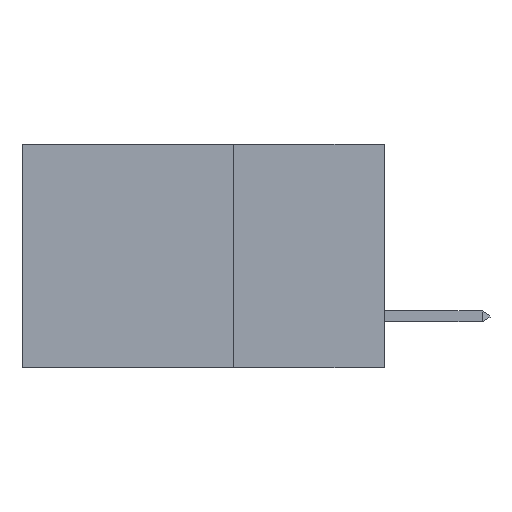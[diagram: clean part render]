
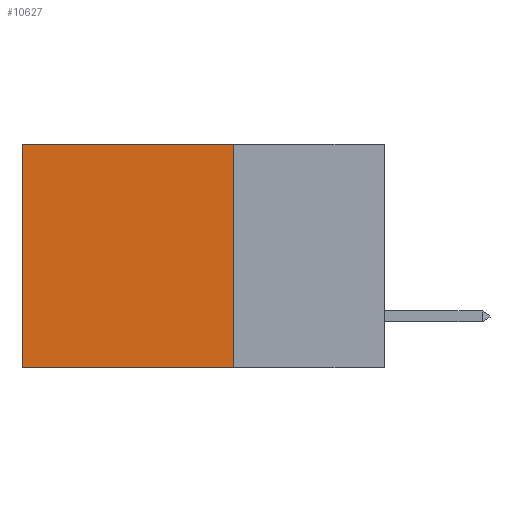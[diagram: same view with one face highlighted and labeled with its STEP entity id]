
A CAD part, left-side view. The second image highlights one B-rep face of the part: STEP entity #10627.
In plain terms, the highlighted planar face has unit normal (-1, 0, 0).
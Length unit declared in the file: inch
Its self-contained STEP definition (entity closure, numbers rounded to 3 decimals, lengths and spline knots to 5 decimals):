
#1636 = DIRECTION ( 'NONE',  ( 0., 0., -1. ) ) ;
#2250 = LINE ( 'NONE', #33708, #26084 ) ;
#4461 = EDGE_CURVE ( 'NONE', #18445, #30422, #2250, .T. ) ;
#4537 = ORIENTED_EDGE ( 'NONE', *, *, #19035, .T. ) ;
#8323 = CARTESIAN_POINT ( 'NONE',  ( 0.2875, 0.6, 0. ) ) ;
#9995 = DIRECTION ( 'NONE',  ( 0., 0., -1. ) ) ;
#10439 = EDGE_CURVE ( 'NONE', #30422, #24059, #21062, .T. ) ;
#10545 = PLANE ( 'NONE',  #28321 ) ;
#10627 = ADVANCED_FACE ( 'NONE', ( #14485 ), #10545, .F. ) ;
#12079 = ORIENTED_EDGE ( 'NONE', *, *, #4461, .F. ) ;
#12773 = DIRECTION ( 'NONE',  ( 0., 1., 0. ) ) ;
#12940 = EDGE_CURVE ( 'NONE', #21688, #24059, #29257, .T. ) ;
#14485 = FACE_OUTER_BOUND ( 'NONE', #36721, .T. ) ;
#15905 = ORIENTED_EDGE ( 'NONE', *, *, #12940, .T. ) ;
#18445 = VERTEX_POINT ( 'NONE', #25985 ) ;
#18540 = ORIENTED_EDGE ( 'NONE', *, *, #10439, .F. ) ;
#19035 = EDGE_CURVE ( 'NONE', #18445, #21688, #29015, .T. ) ;
#19536 = DIRECTION ( 'NONE',  ( 1., 0., 0. ) ) ;
#20107 = VECTOR ( 'NONE', #12773, 39.37008 ) ;
#20172 = VECTOR ( 'NONE', #37490, 39.37008 ) ;
#21062 = LINE ( 'NONE', #30570, #20107 ) ;
#21688 = VERTEX_POINT ( 'NONE', #36506 ) ;
#22385 = CARTESIAN_POINT ( 'NONE',  ( 0.2875, 0.25, -0.37 ) ) ;
#24059 = VERTEX_POINT ( 'NONE', #31439 ) ;
#25812 = CARTESIAN_POINT ( 'NONE',  ( 0.2875, 0.25, 0. ) ) ;
#25985 = CARTESIAN_POINT ( 'NONE',  ( 0.2875, 0.25, 0. ) ) ;
#26084 = VECTOR ( 'NONE', #9995, 39.37008 ) ;
#28321 = AXIS2_PLACEMENT_3D ( 'NONE', #37211, #19536, #1636 ) ;
#29015 = LINE ( 'NONE', #25812, #20172 ) ;
#29257 = LINE ( 'NONE', #8323, #35168 ) ;
#30422 = VERTEX_POINT ( 'NONE', #22385 ) ;
#30570 = CARTESIAN_POINT ( 'NONE',  ( 0.2875, 0.25, -0.37 ) ) ;
#31439 = CARTESIAN_POINT ( 'NONE',  ( 0.2875, 0.6, -0.37 ) ) ;
#31966 = DIRECTION ( 'NONE',  ( 0., 0., -1. ) ) ;
#33708 = CARTESIAN_POINT ( 'NONE',  ( 0.2875, 0.25, 0. ) ) ;
#35168 = VECTOR ( 'NONE', #31966, 39.37008 ) ;
#36506 = CARTESIAN_POINT ( 'NONE',  ( 0.2875, 0.6, 0. ) ) ;
#36721 = EDGE_LOOP ( 'NONE', ( #15905, #18540, #12079, #4537 ) ) ;
#37211 = CARTESIAN_POINT ( 'NONE',  ( 0.2875, 0.25, 0. ) ) ;
#37490 = DIRECTION ( 'NONE',  ( 0., 1., 0. ) ) ;
